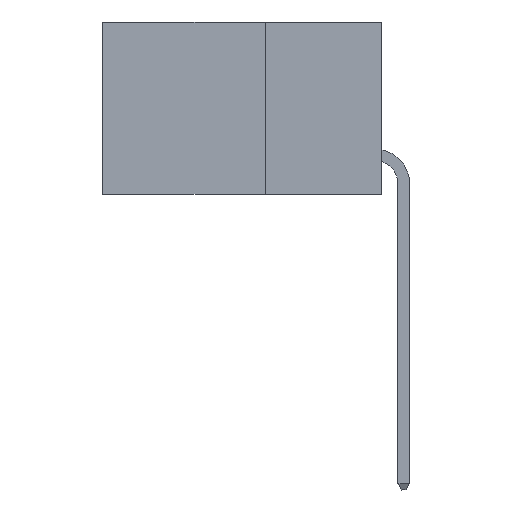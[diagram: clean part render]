
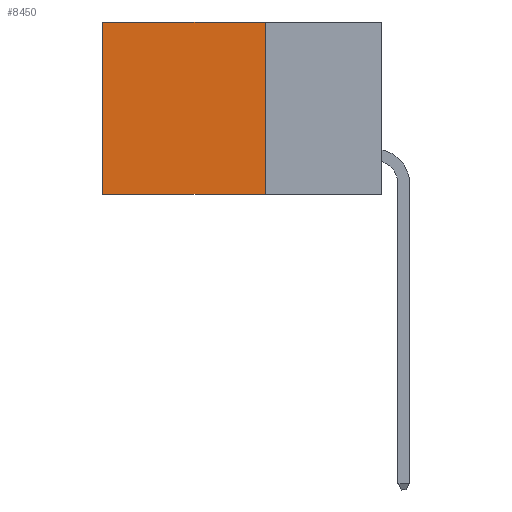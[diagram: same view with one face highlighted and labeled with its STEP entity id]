
A CAD part, left-side view. The second image highlights one B-rep face of the part: STEP entity #8450.
In plain terms, the highlighted planar face has unit normal (-1, 0, 0).
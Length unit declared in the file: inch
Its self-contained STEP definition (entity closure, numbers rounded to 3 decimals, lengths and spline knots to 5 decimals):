
#715 = DIRECTION ( 'NONE',  ( 1., 0., 0. ) ) ;
#3739 = VECTOR ( 'NONE', #31268, 39.37008 ) ;
#7163 = EDGE_CURVE ( 'NONE', #17412, #29693, #27822, .T. ) ;
#8207 = EDGE_CURVE ( 'NONE', #36567, #18601, #13116, .T. ) ;
#8450 = ADVANCED_FACE ( 'NONE', ( #27714 ), #15760, .F. ) ;
#9929 = CARTESIAN_POINT ( 'NONE',  ( 0.2875, 0.25, 0. ) ) ;
#11535 = CARTESIAN_POINT ( 'NONE',  ( 0.2875, 0.25, 0. ) ) ;
#13116 = LINE ( 'NONE', #35678, #36219 ) ;
#15111 = ORIENTED_EDGE ( 'NONE', *, *, #18190, .T. ) ;
#15760 = PLANE ( 'NONE',  #18313 ) ;
#17412 = VERTEX_POINT ( 'NONE', #33453 ) ;
#17721 = VECTOR ( 'NONE', #31024, 39.37008 ) ;
#17783 = CARTESIAN_POINT ( 'NONE',  ( 0.2875, 0.25, -0.37 ) ) ;
#18190 = EDGE_CURVE ( 'NONE', #36567, #17412, #32843, .T. ) ;
#18313 = AXIS2_PLACEMENT_3D ( 'NONE', #36845, #715, #21759 ) ;
#18601 = VERTEX_POINT ( 'NONE', #17783 ) ;
#19042 = LINE ( 'NONE', #27335, #34147 ) ;
#21759 = DIRECTION ( 'NONE',  ( 0., 0., -1. ) ) ;
#21789 = EDGE_LOOP ( 'NONE', ( #34151, #30411, #30216, #15111 ) ) ;
#27335 = CARTESIAN_POINT ( 'NONE',  ( 0.2875, 0.25, -0.37 ) ) ;
#27714 = FACE_OUTER_BOUND ( 'NONE', #21789, .T. ) ;
#27822 = LINE ( 'NONE', #28249, #3739 ) ;
#28249 = CARTESIAN_POINT ( 'NONE',  ( 0.2875, 0.6, 0. ) ) ;
#29693 = VERTEX_POINT ( 'NONE', #35859 ) ;
#29758 = DIRECTION ( 'NONE',  ( 0., 0., -1. ) ) ;
#30216 = ORIENTED_EDGE ( 'NONE', *, *, #8207, .F. ) ;
#30366 = DIRECTION ( 'NONE',  ( 0., 1., 0. ) ) ;
#30411 = ORIENTED_EDGE ( 'NONE', *, *, #34875, .F. ) ;
#31024 = DIRECTION ( 'NONE',  ( 0., 1., 0. ) ) ;
#31268 = DIRECTION ( 'NONE',  ( 0., 0., -1. ) ) ;
#32843 = LINE ( 'NONE', #9929, #17721 ) ;
#33453 = CARTESIAN_POINT ( 'NONE',  ( 0.2875, 0.6, 0. ) ) ;
#34147 = VECTOR ( 'NONE', #30366, 39.37008 ) ;
#34151 = ORIENTED_EDGE ( 'NONE', *, *, #7163, .T. ) ;
#34875 = EDGE_CURVE ( 'NONE', #18601, #29693, #19042, .T. ) ;
#35678 = CARTESIAN_POINT ( 'NONE',  ( 0.2875, 0.25, 0. ) ) ;
#35859 = CARTESIAN_POINT ( 'NONE',  ( 0.2875, 0.6, -0.37 ) ) ;
#36219 = VECTOR ( 'NONE', #29758, 39.37008 ) ;
#36567 = VERTEX_POINT ( 'NONE', #11535 ) ;
#36845 = CARTESIAN_POINT ( 'NONE',  ( 0.2875, 0.25, 0. ) ) ;
